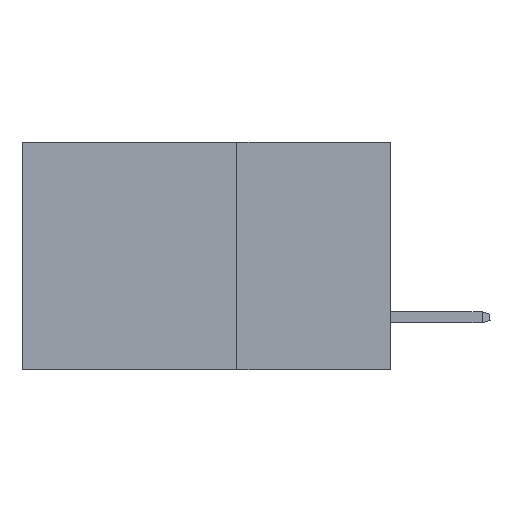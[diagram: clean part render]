
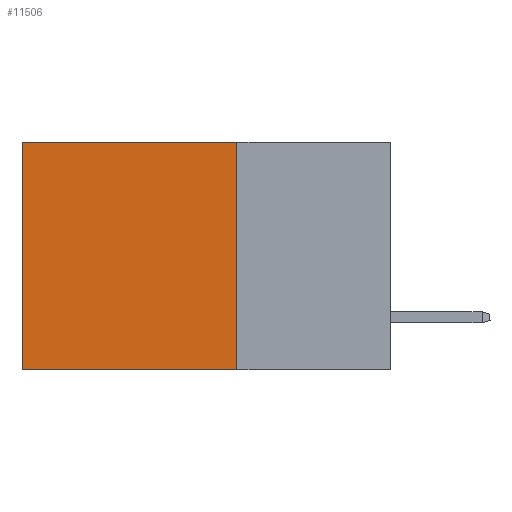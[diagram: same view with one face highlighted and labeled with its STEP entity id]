
A CAD part, left-side view. The second image highlights one B-rep face of the part: STEP entity #11506.
In plain terms, the highlighted planar face has unit normal (-1, 0, 0).
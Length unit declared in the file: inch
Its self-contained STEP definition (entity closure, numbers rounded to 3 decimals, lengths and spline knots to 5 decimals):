
#244 = VERTEX_POINT ( 'NONE', #28838 ) ;
#399 = VECTOR ( 'NONE', #26689, 39.37008 ) ;
#773 = VECTOR ( 'NONE', #1775, 39.37008 ) ;
#1775 = DIRECTION ( 'NONE',  ( 0., 1., 0. ) ) ;
#3177 = PLANE ( 'NONE',  #3316 ) ;
#3316 = AXIS2_PLACEMENT_3D ( 'NONE', #25006, #28118, #9490 ) ;
#5495 = VECTOR ( 'NONE', #26480, 39.37008 ) ;
#8086 = CARTESIAN_POINT ( 'NONE',  ( 0.2875, 0.25, -0.37 ) ) ;
#8221 = CARTESIAN_POINT ( 'NONE',  ( 0.2875, 0.6, 0. ) ) ;
#9005 = CARTESIAN_POINT ( 'NONE',  ( 0.2875, 0.25, -0.37 ) ) ;
#9490 = DIRECTION ( 'NONE',  ( 0., 0., -1. ) ) ;
#9770 = VERTEX_POINT ( 'NONE', #19548 ) ;
#10060 = LINE ( 'NONE', #17181, #773 ) ;
#11506 = ADVANCED_FACE ( 'NONE', ( #22698 ), #3177, .F. ) ;
#15523 = VERTEX_POINT ( 'NONE', #24357 ) ;
#17160 = ORIENTED_EDGE ( 'NONE', *, *, #38298, .F. ) ;
#17181 = CARTESIAN_POINT ( 'NONE',  ( 0.2875, 0.25, 0. ) ) ;
#19548 = CARTESIAN_POINT ( 'NONE',  ( 0.2875, 0.6, 0. ) ) ;
#20664 = DIRECTION ( 'NONE',  ( 0., 0., -1. ) ) ;
#20899 = EDGE_CURVE ( 'NONE', #244, #9770, #10060, .T. ) ;
#21139 = LINE ( 'NONE', #8221, #36627 ) ;
#22698 = FACE_OUTER_BOUND ( 'NONE', #31709, .T. ) ;
#23079 = LINE ( 'NONE', #8086, #5495 ) ;
#23594 = CARTESIAN_POINT ( 'NONE',  ( 0.2875, 0.25, 0. ) ) ;
#24357 = CARTESIAN_POINT ( 'NONE',  ( 0.2875, 0.6, -0.37 ) ) ;
#25006 = CARTESIAN_POINT ( 'NONE',  ( 0.2875, 0.25, 0. ) ) ;
#25255 = LINE ( 'NONE', #23594, #399 ) ;
#26480 = DIRECTION ( 'NONE',  ( 0., 1., 0. ) ) ;
#26689 = DIRECTION ( 'NONE',  ( 0., 0., -1. ) ) ;
#27552 = EDGE_CURVE ( 'NONE', #32396, #15523, #23079, .T. ) ;
#27588 = EDGE_CURVE ( 'NONE', #9770, #15523, #21139, .T. ) ;
#28118 = DIRECTION ( 'NONE',  ( 1., 0., 0. ) ) ;
#28838 = CARTESIAN_POINT ( 'NONE',  ( 0.2875, 0.25, 0. ) ) ;
#31709 = EDGE_LOOP ( 'NONE', ( #35988, #32864, #17160, #32921 ) ) ;
#32396 = VERTEX_POINT ( 'NONE', #9005 ) ;
#32864 = ORIENTED_EDGE ( 'NONE', *, *, #27552, .F. ) ;
#32921 = ORIENTED_EDGE ( 'NONE', *, *, #20899, .T. ) ;
#35988 = ORIENTED_EDGE ( 'NONE', *, *, #27588, .T. ) ;
#36627 = VECTOR ( 'NONE', #20664, 39.37008 ) ;
#38298 = EDGE_CURVE ( 'NONE', #244, #32396, #25255, .T. ) ;
